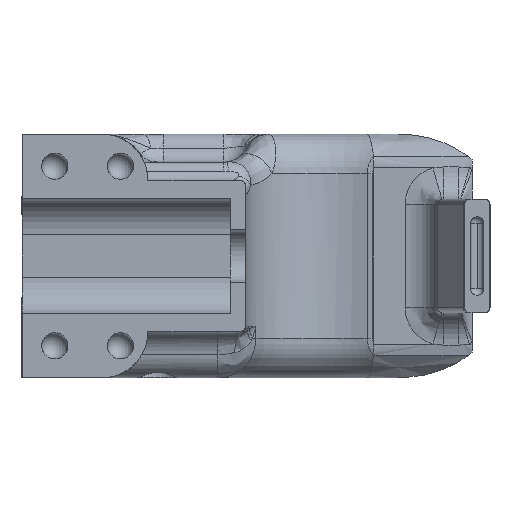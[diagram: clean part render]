
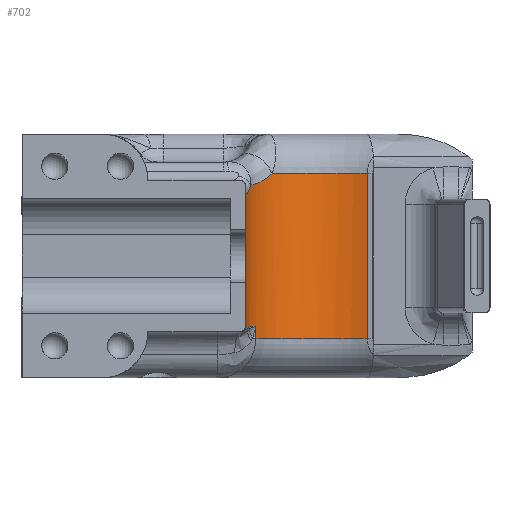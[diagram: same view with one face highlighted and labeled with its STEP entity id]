
A CAD part, front view. The second image highlights one B-rep face of the part: STEP entity #702.
In plain terms, the highlighted cylindrical face has radius 14.287 mm (diameter 28.575 mm), a partial arc.
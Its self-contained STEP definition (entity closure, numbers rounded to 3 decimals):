
#105 = AXIS2_PLACEMENT_3D ( 'NONE', #2241, #7680, #3040 ) ;
#130 = VERTEX_POINT ( 'NONE', #6376 ) ;
#149 = ORIENTED_EDGE ( 'NONE', *, *, #9904, .F. ) ;
#272 = CARTESIAN_POINT ( 'NONE',  ( 35.117, -179.957, 15.378 ) ) ;
#309 = CARTESIAN_POINT ( 'NONE',  ( 34.358, -183.685, 14.259 ) ) ;
#424 = CARTESIAN_POINT ( 'NONE',  ( 52.867, -171., -9.74 ) ) ;
#442 = DIRECTION ( 'NONE',  ( 0., 1., 0. ) ) ;
#462 = VERTEX_POINT ( 'NONE', #5221 ) ;
#541 = DIRECTION ( 'NONE',  ( 0., 0., -1. ) ) ;
#699 = EDGE_CURVE ( 'NONE', #3895, #8602, #7434, .T. ) ;
#702 = ADVANCED_FACE ( 'NONE', ( #9230 ), #1013, .F. ) ;
#1013 = CYLINDRICAL_SURFACE ( 'NONE', #9871, 14.288 ) ;
#1049 = CARTESIAN_POINT ( 'NONE',  ( 35.023, -180.23, 15.032 ) ) ;
#1084 = CARTESIAN_POINT ( 'NONE',  ( 34.331, -184.279, 14.56 ) ) ;
#1139 = CARTESIAN_POINT ( 'NONE',  ( 34.789, -181.042, -6.168 ) ) ;
#1188 = ORIENTED_EDGE ( 'NONE', *, *, #4921, .F. ) ;
#1424 = VERTEX_POINT ( 'NONE', #4866 ) ;
#1533 = EDGE_CURVE ( 'NONE', #8602, #4415, #5347, .T. ) ;
#1646 = CARTESIAN_POINT ( 'NONE',  ( 37.742, -175.359, 16.517 ) ) ;
#1819 = CARTESIAN_POINT ( 'NONE',  ( 34.92, -180.553, 14.742 ) ) ;
#1853 = CARTESIAN_POINT ( 'NONE',  ( 34.328, -184.64, 14.834 ) ) ;
#1864 = CARTESIAN_POINT ( 'NONE',  ( 35.912, -178.102, -6.168 ) ) ;
#2009 = ORIENTED_EDGE ( 'NONE', *, *, #4764, .T. ) ;
#2160 = LINE ( 'NONE', #424, #9184 ) ;
#2217 = VERTEX_POINT ( 'NONE', #1139 ) ;
#2241 = CARTESIAN_POINT ( 'NONE',  ( 48.616, -184.64, -6.168 ) ) ;
#2409 = CARTESIAN_POINT ( 'NONE',  ( 36.807, -176.579, 15.909 ) ) ;
#2548 = B_SPLINE_CURVE_WITH_KNOTS ( 'NONE', 3,
 ( #5499, #7805, #1646, #7066, #2409, #7836, #3203, #8601, #3982, #9377 ),
 .UNSPECIFIED., .F., .F.,
 ( 4, 2, 2, 2, 4 ),
 ( 0., 0.002, 0.003, 0.005, 0.007 ),
 .UNSPECIFIED. ) ;
#2593 = CARTESIAN_POINT ( 'NONE',  ( 34.719, -181.314, 14.31 ) ) ;
#2825 = DIRECTION ( 'NONE',  ( 0., 1., 0. ) ) ;
#2830 = ORIENTED_EDGE ( 'NONE', *, *, #1533, .T. ) ;
#2890 = ORIENTED_EDGE ( 'NONE', *, *, #9272, .T. ) ;
#2987 = CARTESIAN_POINT ( 'NONE',  ( 48.616, -184.64, 17.114 ) ) ;
#3040 = DIRECTION ( 'NONE',  ( 0., 1., 0. ) ) ;
#3203 = CARTESIAN_POINT ( 'NONE',  ( 35.973, -177.963, 15.564 ) ) ;
#3377 = CARTESIAN_POINT ( 'NONE',  ( 34.584, -181.938, 14.112 ) ) ;
#3609 = CARTESIAN_POINT ( 'NONE',  ( 35.912, -178.102, -9.74 ) ) ;
#3768 = DIRECTION ( 'NONE',  ( 0., 1., 0. ) ) ;
#3895 = VERTEX_POINT ( 'NONE', #1864 ) ;
#3982 = CARTESIAN_POINT ( 'NONE',  ( 35.297, -179.44, 15.401 ) ) ;
#4161 = CARTESIAN_POINT ( 'NONE',  ( 34.473, -182.597, 14.049 ) ) ;
#4178 = B_SPLINE_CURVE_WITH_KNOTS ( 'NONE', 3,
 ( #272, #1049, #1819, #7241, #2593, #8004, #3377, #8782, #4161, #9556, #4931, #309, #5700, #1084, #6491, #1853 ),
 .UNSPECIFIED., .F., .F.,
 ( 4, 2, 2, 2, 2, 2, 2, 4 ),
 ( 0., 0.001, 0.002, 0.003, 0.003, 0.004, 0.005, 0.005 ),
 .UNSPECIFIED. ) ;
#4223 = LINE ( 'NONE', #8763, #7850 ) ;
#4233 = DIRECTION ( 'NONE',  ( 0., 0., -1. ) ) ;
#4415 = VERTEX_POINT ( 'NONE', #8043 ) ;
#4764 = EDGE_CURVE ( 'NONE', #2217, #3895, #9097, .T. ) ;
#4866 = CARTESIAN_POINT ( 'NONE',  ( 52.867, -171., 17.114 ) ) ;
#4921 = EDGE_CURVE ( 'NONE', #2217, #462, #5827, .T. ) ;
#4931 = CARTESIAN_POINT ( 'NONE',  ( 34.393, -183.258, 14.128 ) ) ;
#4992 = VERTEX_POINT ( 'NONE', #6924 ) ;
#5070 = DIRECTION ( 'NONE',  ( 0., 0., -1. ) ) ;
#5077 = DIRECTION ( 'NONE',  ( 0., 0., 1. ) ) ;
#5207 = ORIENTED_EDGE ( 'NONE', *, *, #699, .T. ) ;
#5221 = CARTESIAN_POINT ( 'NONE',  ( 34.328, -184.64, -6.168 ) ) ;
#5347 = CIRCLE ( 'NONE', #9283, 14.288 ) ;
#5499 = CARTESIAN_POINT ( 'NONE',  ( 38.372, -174.68, 17.114 ) ) ;
#5615 = EDGE_CURVE ( 'NONE', #1424, #4992, #9686, .T. ) ;
#5700 = CARTESIAN_POINT ( 'NONE',  ( 34.346, -183.889, 14.346 ) ) ;
#5707 = ORIENTED_EDGE ( 'NONE', *, *, #7778, .T. ) ;
#5827 = CIRCLE ( 'NONE', #105, 14.288 ) ;
#5848 = EDGE_CURVE ( 'NONE', #7393, #130, #4178, .T. ) ;
#5928 = CARTESIAN_POINT ( 'NONE',  ( 48.616, -184.64, -9.74 ) ) ;
#6120 = ORIENTED_EDGE ( 'NONE', *, *, #5848, .T. ) ;
#6226 = ORIENTED_EDGE ( 'NONE', *, *, #5615, .T. ) ;
#6376 = CARTESIAN_POINT ( 'NONE',  ( 34.328, -184.64, 14.834 ) ) ;
#6468 = AXIS2_PLACEMENT_3D ( 'NONE', #2987, #8385, #3768 ) ;
#6491 = CARTESIAN_POINT ( 'NONE',  ( 34.328, -184.467, 14.689 ) ) ;
#6525 = AXIS2_PLACEMENT_3D ( 'NONE', #9691, #5070, #442 ) ;
#6924 = CARTESIAN_POINT ( 'NONE',  ( 38.372, -174.68, 17.114 ) ) ;
#7066 = CARTESIAN_POINT ( 'NONE',  ( 37.117, -176.145, 16.079 ) ) ;
#7163 = CARTESIAN_POINT ( 'NONE',  ( 35.912, -178.102, -8.019 ) ) ;
#7241 = CARTESIAN_POINT ( 'NONE',  ( 34.768, -181.118, 14.403 ) ) ;
#7322 = DIRECTION ( 'NONE',  ( 0., 0., 1. ) ) ;
#7393 = VERTEX_POINT ( 'NONE', #7642 ) ;
#7434 = LINE ( 'NONE', #3609, #9463 ) ;
#7498 = DIRECTION ( 'NONE',  ( 0., 0., 1. ) ) ;
#7642 = CARTESIAN_POINT ( 'NONE',  ( 35.117, -179.957, 15.378 ) ) ;
#7680 = DIRECTION ( 'NONE',  ( 0., 0., 1. ) ) ;
#7778 = EDGE_CURVE ( 'NONE', #4992, #7393, #2548, .T. ) ;
#7805 = CARTESIAN_POINT ( 'NONE',  ( 38.059, -175.002, 16.784 ) ) ;
#7836 = CARTESIAN_POINT ( 'NONE',  ( 36.234, -177.491, 15.651 ) ) ;
#7850 = VECTOR ( 'NONE', #7322, 1000. ) ;
#8004 = CARTESIAN_POINT ( 'NONE',  ( 34.627, -181.723, 14.165 ) ) ;
#8043 = CARTESIAN_POINT ( 'NONE',  ( 52.867, -171., -8.019 ) ) ;
#8233 = EDGE_LOOP ( 'NONE', ( #5707, #6120, #149, #1188, #2009, #5207, #2830, #2890, #6226 ) ) ;
#8385 = DIRECTION ( 'NONE',  ( 0., 0., 1. ) ) ;
#8601 = CARTESIAN_POINT ( 'NONE',  ( 35.504, -178.938, 15.439 ) ) ;
#8602 = VERTEX_POINT ( 'NONE', #7163 ) ;
#8763 = CARTESIAN_POINT ( 'NONE',  ( 34.328, -184.64, -9.74 ) ) ;
#8782 = CARTESIAN_POINT ( 'NONE',  ( 34.507, -182.377, 14.054 ) ) ;
#8854 = CARTESIAN_POINT ( 'NONE',  ( 48.616, -184.64, -8.019 ) ) ;
#9097 = CIRCLE ( 'NONE', #6525, 14.288 ) ;
#9184 = VECTOR ( 'NONE', #5077, 1000. ) ;
#9230 = FACE_OUTER_BOUND ( 'NONE', #8233, .T. ) ;
#9272 = EDGE_CURVE ( 'NONE', #4415, #1424, #2160, .T. ) ;
#9283 = AXIS2_PLACEMENT_3D ( 'NONE', #8854, #4233, #9637 ) ;
#9377 = CARTESIAN_POINT ( 'NONE',  ( 35.117, -179.957, 15.378 ) ) ;
#9463 = VECTOR ( 'NONE', #541, 1000. ) ;
#9556 = CARTESIAN_POINT ( 'NONE',  ( 34.417, -183.036, 14.086 ) ) ;
#9637 = DIRECTION ( 'NONE',  ( 0., 1., 0. ) ) ;
#9686 = CIRCLE ( 'NONE', #6468, 14.288 ) ;
#9691 = CARTESIAN_POINT ( 'NONE',  ( 48.616, -184.64, -6.168 ) ) ;
#9871 = AXIS2_PLACEMENT_3D ( 'NONE', #5928, #7498, #2825 ) ;
#9904 = EDGE_CURVE ( 'NONE', #462, #130, #4223, .T. ) ;
